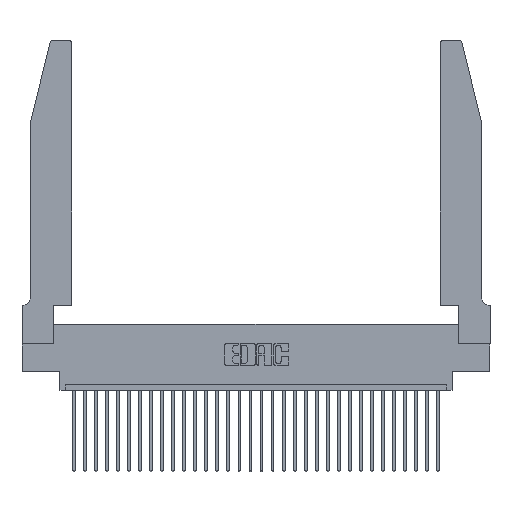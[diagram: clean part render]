
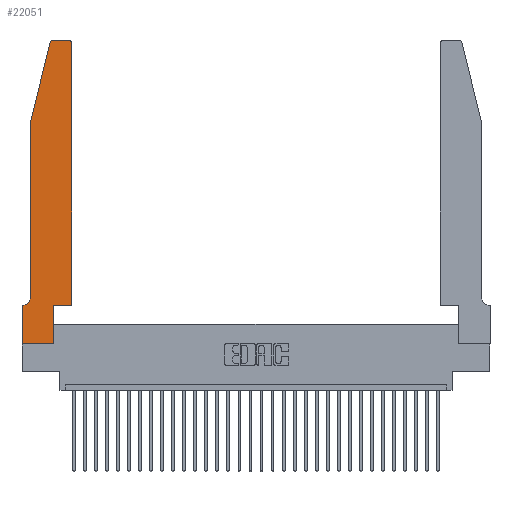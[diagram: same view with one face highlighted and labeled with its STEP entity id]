
A CAD part, top view. The second image highlights one B-rep face of the part: STEP entity #22051.
In plain terms, the highlighted planar face has unit normal (0, 0, 1).
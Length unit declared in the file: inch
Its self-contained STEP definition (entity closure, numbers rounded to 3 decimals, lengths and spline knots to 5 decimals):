
#362 = EDGE_CURVE ( 'NONE', #27027, #1338, #18498, .T. ) ;
#793 = CARTESIAN_POINT ( 'NONE',  ( 0.0755, 2., 0.37 ) ) ;
#1115 = LINE ( 'NONE', #28187, #27830 ) ;
#1186 = DIRECTION ( 'NONE',  ( 1., 0., 0. ) ) ;
#1338 = VERTEX_POINT ( 'NONE', #4147 ) ;
#1604 = CIRCLE ( 'NONE', #11642, 0.07 ) ;
#1912 = DIRECTION ( 'NONE',  ( 0., 1., 0. ) ) ;
#2114 = CARTESIAN_POINT ( 'NONE',  ( 0.4505, 0.35, 0.37 ) ) ;
#2554 = CARTESIAN_POINT ( 'NONE',  ( 0.25487, 2.72718, 0.37 ) ) ;
#3260 = EDGE_CURVE ( 'NONE', #4135, #20988, #4236, .T. ) ;
#3483 = CARTESIAN_POINT ( 'NONE',  ( 0., 0.35, 0.37 ) ) ;
#3534 = EDGE_CURVE ( 'NONE', #29808, #4135, #1115, .T. ) ;
#3809 = LINE ( 'NONE', #793, #8085 ) ;
#3918 = CARTESIAN_POINT ( 'NONE',  ( 0.0755, 2., 0.37 ) ) ;
#4063 = CARTESIAN_POINT ( 'NONE',  ( 0.2865, 0.35, 0.37 ) ) ;
#4135 = VERTEX_POINT ( 'NONE', #29401 ) ;
#4147 = CARTESIAN_POINT ( 'NONE',  ( 0.284, 2.75, 0.37 ) ) ;
#4188 = CARTESIAN_POINT ( 'NONE',  ( 0., 0., 0.37 ) ) ;
#4236 = LINE ( 'NONE', #4188, #21021 ) ;
#4809 = VERTEX_POINT ( 'NONE', #2554 ) ;
#5219 = CARTESIAN_POINT ( 'NONE',  ( 0.0055, 0.35, 0.37 ) ) ;
#5455 = ORIENTED_EDGE ( 'NONE', *, *, #23253, .T. ) ;
#5735 = VERTEX_POINT ( 'NONE', #5219 ) ;
#5756 = CARTESIAN_POINT ( 'NONE',  ( 0.4205, 2.75, 0.37 ) ) ;
#6186 = VECTOR ( 'NONE', #15049, 39.37008 ) ;
#6438 = ORIENTED_EDGE ( 'NONE', *, *, #8199, .T. ) ;
#6454 = ORIENTED_EDGE ( 'NONE', *, *, #3534, .T. ) ;
#6629 = ORIENTED_EDGE ( 'NONE', *, *, #11596, .T. ) ;
#6857 = DIRECTION ( 'NONE',  ( -0.239, -0.971, 0. ) ) ;
#7880 = CIRCLE ( 'NONE', #8791, 0.03 ) ;
#8036 = VECTOR ( 'NONE', #21916, 39.37008 ) ;
#8085 = VECTOR ( 'NONE', #16084, 39.37008 ) ;
#8199 = EDGE_CURVE ( 'NONE', #20988, #24148, #29475, .T. ) ;
#8260 = DIRECTION ( 'NONE',  ( 0., 0., 1. ) ) ;
#8469 = DIRECTION ( 'NONE',  ( 1., 0., 0. ) ) ;
#8791 = AXIS2_PLACEMENT_3D ( 'NONE', #19107, #16687, #23996 ) ;
#8799 = LINE ( 'NONE', #19043, #8036 ) ;
#8955 = VERTEX_POINT ( 'NONE', #17484 ) ;
#9504 = CARTESIAN_POINT ( 'NONE',  ( 0.2605, 2.75, 0.37 ) ) ;
#9707 = VECTOR ( 'NONE', #29257, 39.37008 ) ;
#9907 = ORIENTED_EDGE ( 'NONE', *, *, #3260, .T. ) ;
#10074 = CARTESIAN_POINT ( 'NONE',  ( 0., 0.35, 0.37 ) ) ;
#11596 = EDGE_CURVE ( 'NONE', #5735, #29808, #8799, .T. ) ;
#11642 = AXIS2_PLACEMENT_3D ( 'NONE', #26517, #29068, #17190 ) ;
#11906 = VERTEX_POINT ( 'NONE', #16580 ) ;
#12287 = CARTESIAN_POINT ( 'NONE',  ( 0.4505, 0.35, 0.37 ) ) ;
#12338 = LINE ( 'NONE', #12287, #9707 ) ;
#12685 = LINE ( 'NONE', #29619, #6186 ) ;
#13034 = PLANE ( 'NONE',  #22048 ) ;
#13374 = VERTEX_POINT ( 'NONE', #2114 ) ;
#15049 = DIRECTION ( 'NONE',  ( 0., 1., 0. ) ) ;
#16043 = ORIENTED_EDGE ( 'NONE', *, *, #22770, .T. ) ;
#16084 = DIRECTION ( 'NONE',  ( 0., -1., 0. ) ) ;
#16523 = VECTOR ( 'NONE', #6857, 39.37008 ) ;
#16580 = CARTESIAN_POINT ( 'NONE',  ( 0.0755, 0.42, 0.37 ) ) ;
#16687 = DIRECTION ( 'NONE',  ( 0., 0., 1. ) ) ;
#17190 = DIRECTION ( 'NONE',  ( -1., 0., 0. ) ) ;
#17484 = CARTESIAN_POINT ( 'NONE',  ( 0.4505, 2.72, 0.37 ) ) ;
#18498 = LINE ( 'NONE', #9504, #30643 ) ;
#19043 = CARTESIAN_POINT ( 'NONE',  ( 0.0755, 0.35, 0.37 ) ) ;
#19107 = CARTESIAN_POINT ( 'NONE',  ( 0.4205, 2.72, 0.37 ) ) ;
#19268 = ORIENTED_EDGE ( 'NONE', *, *, #22556, .T. ) ;
#20528 = CARTESIAN_POINT ( 'NONE',  ( 0.284, 2.72, 0.37 ) ) ;
#20556 = EDGE_CURVE ( 'NONE', #8955, #27027, #7880, .T. ) ;
#20557 = EDGE_CURVE ( 'NONE', #11906, #5735, #1604, .T. ) ;
#20875 = EDGE_LOOP ( 'NONE', ( #26769, #23731, #19268, #5455, #29456, #6629, #6454, #9907, #6438, #27154, #16043, #21328 ) ) ;
#20988 = VERTEX_POINT ( 'NONE', #29289 ) ;
#21021 = VECTOR ( 'NONE', #21244, 39.37008 ) ;
#21244 = DIRECTION ( 'NONE',  ( 1., 0., 0. ) ) ;
#21328 = ORIENTED_EDGE ( 'NONE', *, *, #20556, .T. ) ;
#21515 = EDGE_CURVE ( 'NONE', #1338, #4809, #30193, .T. ) ;
#21916 = DIRECTION ( 'NONE',  ( -1., 0., 0. ) ) ;
#22048 = AXIS2_PLACEMENT_3D ( 'NONE', #3483, #8260, #8469 ) ;
#22051 = ADVANCED_FACE ( 'NONE', ( #26389 ), #13034, .T. ) ;
#22371 = EDGE_CURVE ( 'NONE', #24148, #13374, #12338, .T. ) ;
#22556 = EDGE_CURVE ( 'NONE', #4809, #29965, #22947, .T. ) ;
#22569 = CARTESIAN_POINT ( 'NONE',  ( 0.2865, 0.35, 0.37 ) ) ;
#22770 = EDGE_CURVE ( 'NONE', #13374, #8955, #12685, .T. ) ;
#22947 = LINE ( 'NONE', #3918, #16523 ) ;
#23007 = VECTOR ( 'NONE', #1912, 39.37008 ) ;
#23253 = EDGE_CURVE ( 'NONE', #29965, #11906, #3809, .T. ) ;
#23731 = ORIENTED_EDGE ( 'NONE', *, *, #21515, .T. ) ;
#23996 = DIRECTION ( 'NONE',  ( 1., 0., 0. ) ) ;
#24148 = VERTEX_POINT ( 'NONE', #22569 ) ;
#24156 = DIRECTION ( 'NONE',  ( -1., 0., 0. ) ) ;
#24347 = DIRECTION ( 'NONE',  ( 0., -1., 0. ) ) ;
#26389 = FACE_OUTER_BOUND ( 'NONE', #20875, .T. ) ;
#26517 = CARTESIAN_POINT ( 'NONE',  ( 0.0055, 0.42, 0.37 ) ) ;
#26769 = ORIENTED_EDGE ( 'NONE', *, *, #362, .T. ) ;
#27027 = VERTEX_POINT ( 'NONE', #5756 ) ;
#27154 = ORIENTED_EDGE ( 'NONE', *, *, #22371, .T. ) ;
#27830 = VECTOR ( 'NONE', #24347, 39.37008 ) ;
#28187 = CARTESIAN_POINT ( 'NONE',  ( 0., 0., 0.37 ) ) ;
#29068 = DIRECTION ( 'NONE',  ( 0., 0., -1. ) ) ;
#29257 = DIRECTION ( 'NONE',  ( 1., 0., 0. ) ) ;
#29289 = CARTESIAN_POINT ( 'NONE',  ( 0.2865, 0., 0.37 ) ) ;
#29345 = AXIS2_PLACEMENT_3D ( 'NONE', #20528, #30293, #1186 ) ;
#29401 = CARTESIAN_POINT ( 'NONE',  ( 0., 0., 0.37 ) ) ;
#29456 = ORIENTED_EDGE ( 'NONE', *, *, #20557, .T. ) ;
#29475 = LINE ( 'NONE', #4063, #23007 ) ;
#29501 = CARTESIAN_POINT ( 'NONE',  ( 0.0755, 2., 0.37 ) ) ;
#29619 = CARTESIAN_POINT ( 'NONE',  ( 0.4505, 0.35, 0.37 ) ) ;
#29808 = VERTEX_POINT ( 'NONE', #10074 ) ;
#29965 = VERTEX_POINT ( 'NONE', #29501 ) ;
#30193 = CIRCLE ( 'NONE', #29345, 0.03 ) ;
#30293 = DIRECTION ( 'NONE',  ( 0., 0., 1. ) ) ;
#30643 = VECTOR ( 'NONE', #24156, 39.37008 ) ;
